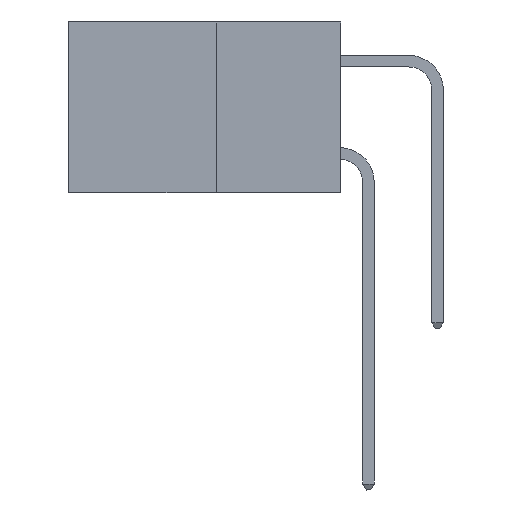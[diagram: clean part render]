
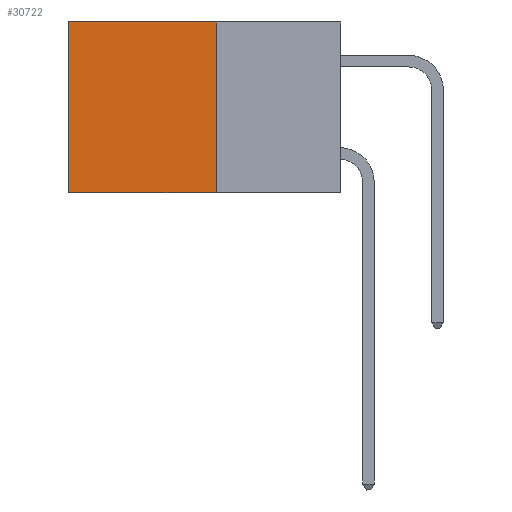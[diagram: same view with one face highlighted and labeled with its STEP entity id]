
A CAD part, left-side view. The second image highlights one B-rep face of the part: STEP entity #30722.
In plain terms, the highlighted planar face has unit normal (-1, 0, 0).
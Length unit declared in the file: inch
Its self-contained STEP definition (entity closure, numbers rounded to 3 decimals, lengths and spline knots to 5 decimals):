
#732 = DIRECTION ( 'NONE',  ( 1., 0., 0. ) ) ;
#981 = VECTOR ( 'NONE', #3772, 39.37008 ) ;
#1150 = LINE ( 'NONE', #21775, #15068 ) ;
#2639 = FACE_OUTER_BOUND ( 'NONE', #28789, .T. ) ;
#3772 = DIRECTION ( 'NONE',  ( 0., 1., 0. ) ) ;
#4544 = CARTESIAN_POINT ( 'NONE',  ( 0.277, 0.27, -0.37 ) ) ;
#7314 = DIRECTION ( 'NONE',  ( 0., 1., 0. ) ) ;
#7494 = LINE ( 'NONE', #4544, #28560 ) ;
#8956 = EDGE_CURVE ( 'NONE', #11089, #10667, #1150, .T. ) ;
#10567 = VECTOR ( 'NONE', #26228, 39.37008 ) ;
#10667 = VERTEX_POINT ( 'NONE', #30672 ) ;
#11089 = VERTEX_POINT ( 'NONE', #34857 ) ;
#13077 = ORIENTED_EDGE ( 'NONE', *, *, #33334, .T. ) ;
#13476 = DIRECTION ( 'NONE',  ( 0., 0., -1. ) ) ;
#14600 = CARTESIAN_POINT ( 'NONE',  ( 0.277, 0.27, -0.37 ) ) ;
#15068 = VECTOR ( 'NONE', #13476, 39.37008 ) ;
#15941 = VERTEX_POINT ( 'NONE', #33396 ) ;
#18244 = EDGE_CURVE ( 'NONE', #10667, #15941, #7494, .T. ) ;
#18736 = LINE ( 'NONE', #23485, #10567 ) ;
#19818 = CARTESIAN_POINT ( 'NONE',  ( 0.277, 0.59, 0. ) ) ;
#20146 = DIRECTION ( 'NONE',  ( 0., 0., -1. ) ) ;
#20311 = CARTESIAN_POINT ( 'NONE',  ( 0.277, 0.27, 0. ) ) ;
#21775 = CARTESIAN_POINT ( 'NONE',  ( 0.277, 0.27, -0.37 ) ) ;
#23485 = CARTESIAN_POINT ( 'NONE',  ( 0.277, 0.59, -0.37 ) ) ;
#24756 = ORIENTED_EDGE ( 'NONE', *, *, #18244, .F. ) ;
#26228 = DIRECTION ( 'NONE',  ( 0., 0., -1. ) ) ;
#26745 = EDGE_CURVE ( 'NONE', #29957, #15941, #18736, .T. ) ;
#28560 = VECTOR ( 'NONE', #7314, 39.37008 ) ;
#28789 = EDGE_LOOP ( 'NONE', ( #29167, #24756, #34508, #13077 ) ) ;
#29167 = ORIENTED_EDGE ( 'NONE', *, *, #26745, .T. ) ;
#29434 = LINE ( 'NONE', #20311, #981 ) ;
#29957 = VERTEX_POINT ( 'NONE', #19818 ) ;
#30080 = AXIS2_PLACEMENT_3D ( 'NONE', #14600, #732, #20146 ) ;
#30672 = CARTESIAN_POINT ( 'NONE',  ( 0.277, 0.27, -0.37 ) ) ;
#30722 = ADVANCED_FACE ( 'NONE', ( #2639 ), #30943, .F. ) ;
#30943 = PLANE ( 'NONE',  #30080 ) ;
#33334 = EDGE_CURVE ( 'NONE', #11089, #29957, #29434, .T. ) ;
#33396 = CARTESIAN_POINT ( 'NONE',  ( 0.277, 0.59, -0.37 ) ) ;
#34508 = ORIENTED_EDGE ( 'NONE', *, *, #8956, .F. ) ;
#34857 = CARTESIAN_POINT ( 'NONE',  ( 0.277, 0.27, 0. ) ) ;
